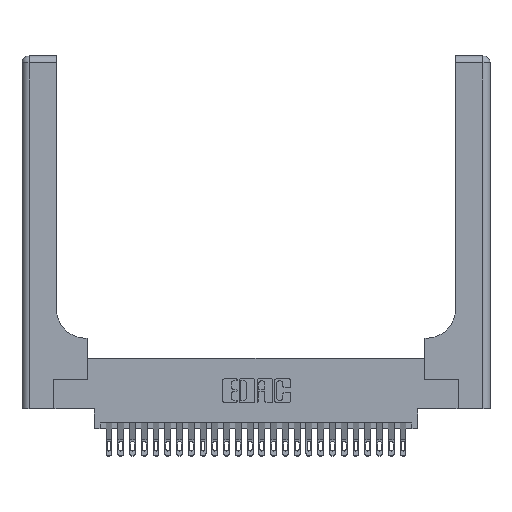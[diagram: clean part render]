
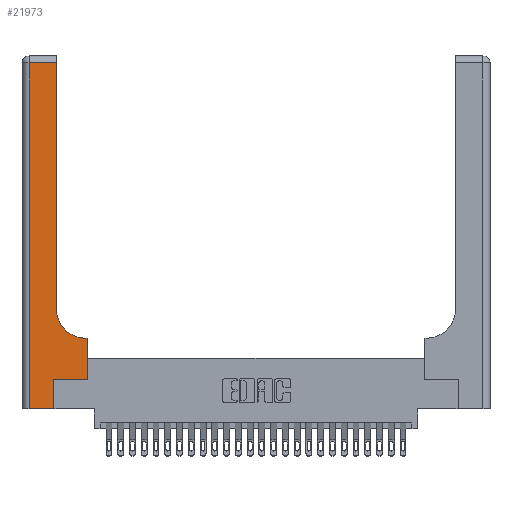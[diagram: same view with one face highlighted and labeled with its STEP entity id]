
A CAD part, top view. The second image highlights one B-rep face of the part: STEP entity #21973.
In plain terms, the highlighted planar face has unit normal (0, 0, 1).
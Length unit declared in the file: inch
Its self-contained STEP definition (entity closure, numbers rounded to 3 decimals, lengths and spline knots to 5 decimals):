
#209 = CARTESIAN_POINT ( 'NONE',  ( 0.269, 0.25, 0.37 ) ) ;
#457 = CARTESIAN_POINT ( 'NONE',  ( 0., 0., 0.37 ) ) ;
#491 = VECTOR ( 'NONE', #25739, 39.37008 ) ;
#656 = CARTESIAN_POINT ( 'NONE',  ( 0., 3., 0.37 ) ) ;
#735 = DIRECTION ( 'NONE',  ( 1., 0., 0. ) ) ;
#740 = DIRECTION ( 'NONE',  ( -1., 0., 0. ) ) ;
#935 = CARTESIAN_POINT ( 'NONE',  ( 0., 2.94, 0.37 ) ) ;
#1166 = LINE ( 'NONE', #1930, #491 ) ;
#1375 = EDGE_CURVE ( 'NONE', #7321, #15064, #19014, .T. ) ;
#1600 = VECTOR ( 'NONE', #14441, 39.37008 ) ;
#1606 = LINE ( 'NONE', #5508, #7385 ) ;
#1655 = EDGE_CURVE ( 'NONE', #11842, #16809, #8755, .T. ) ;
#1930 = CARTESIAN_POINT ( 'NONE',  ( 0.2915, 0.6, 0.37 ) ) ;
#2128 = ORIENTED_EDGE ( 'NONE', *, *, #1655, .T. ) ;
#3147 = ORIENTED_EDGE ( 'NONE', *, *, #14382, .T. ) ;
#3150 = EDGE_CURVE ( 'NONE', #15064, #8248, #1166, .T. ) ;
#3620 = VERTEX_POINT ( 'NONE', #9358 ) ;
#3794 = CARTESIAN_POINT ( 'NONE',  ( 0.2915, 0.85, 0.37 ) ) ;
#3897 = EDGE_CURVE ( 'NONE', #16809, #7321, #12347, .T. ) ;
#5000 = DIRECTION ( 'NONE',  ( 0., 0., -1. ) ) ;
#5508 = CARTESIAN_POINT ( 'NONE',  ( 0.2915, 3., 0.37 ) ) ;
#6095 = ORIENTED_EDGE ( 'NONE', *, *, #3150, .T. ) ;
#6432 = LINE ( 'NONE', #935, #14989 ) ;
#7063 = EDGE_CURVE ( 'NONE', #9543, #10116, #1606, .T. ) ;
#7064 = ORIENTED_EDGE ( 'NONE', *, *, #23813, .T. ) ;
#7321 = VERTEX_POINT ( 'NONE', #18527 ) ;
#7385 = VECTOR ( 'NONE', #20777, 39.37008 ) ;
#7601 = EDGE_LOOP ( 'NONE', ( #12397, #7064, #18103, #3147, #2128, #11591, #24524, #6095, #18890 ) ) ;
#8048 = DIRECTION ( 'NONE',  ( 0., 0., -1. ) ) ;
#8248 = VERTEX_POINT ( 'NONE', #21122 ) ;
#8755 = LINE ( 'NONE', #27491, #1600 ) ;
#9358 = CARTESIAN_POINT ( 'NONE',  ( 0.06, 2.94, 0.37 ) ) ;
#9543 = VERTEX_POINT ( 'NONE', #3794 ) ;
#9610 = VECTOR ( 'NONE', #735, 39.37008 ) ;
#10116 = VERTEX_POINT ( 'NONE', #20019 ) ;
#11130 = CARTESIAN_POINT ( 'NONE',  ( 0.5585, 0.25, 0.37 ) ) ;
#11318 = VERTEX_POINT ( 'NONE', #24661 ) ;
#11519 = CARTESIAN_POINT ( 'NONE',  ( 0.269, 0.25, 0.37 ) ) ;
#11591 = ORIENTED_EDGE ( 'NONE', *, *, #3897, .T. ) ;
#11675 = FACE_OUTER_BOUND ( 'NONE', #7601, .T. ) ;
#11842 = VERTEX_POINT ( 'NONE', #13025 ) ;
#12347 = LINE ( 'NONE', #209, #26332 ) ;
#12397 = ORIENTED_EDGE ( 'NONE', *, *, #7063, .T. ) ;
#12778 = EDGE_CURVE ( 'NONE', #8248, #9543, #13452, .T. ) ;
#13025 = CARTESIAN_POINT ( 'NONE',  ( 0.269, 0., 0.37 ) ) ;
#13452 = CIRCLE ( 'NONE', #27982, 0.25 ) ;
#14382 = EDGE_CURVE ( 'NONE', #11318, #11842, #16123, .T. ) ;
#14441 = DIRECTION ( 'NONE',  ( 0., 1., 0. ) ) ;
#14989 = VECTOR ( 'NONE', #16240, 39.37008 ) ;
#15064 = VERTEX_POINT ( 'NONE', #16015 ) ;
#15498 = VECTOR ( 'NONE', #19671, 39.37008 ) ;
#16015 = CARTESIAN_POINT ( 'NONE',  ( 0.5585, 0.6, 0.37 ) ) ;
#16123 = LINE ( 'NONE', #457, #9610 ) ;
#16240 = DIRECTION ( 'NONE',  ( -1., 0., 0. ) ) ;
#16510 = AXIS2_PLACEMENT_3D ( 'NONE', #656, #5000, #740 ) ;
#16809 = VERTEX_POINT ( 'NONE', #11519 ) ;
#17077 = CARTESIAN_POINT ( 'NONE',  ( 0.5415, 0.85, 0.37 ) ) ;
#17554 = LINE ( 'NONE', #26039, #15498 ) ;
#18103 = ORIENTED_EDGE ( 'NONE', *, *, #21275, .T. ) ;
#18527 = CARTESIAN_POINT ( 'NONE',  ( 0.5585, 0.25, 0.37 ) ) ;
#18890 = ORIENTED_EDGE ( 'NONE', *, *, #12778, .T. ) ;
#19014 = LINE ( 'NONE', #11130, #24116 ) ;
#19181 = DIRECTION ( 'NONE',  ( 1., 0., 0. ) ) ;
#19671 = DIRECTION ( 'NONE',  ( 0., -1., 0. ) ) ;
#20019 = CARTESIAN_POINT ( 'NONE',  ( 0.2915, 2.94, 0.37 ) ) ;
#20777 = DIRECTION ( 'NONE',  ( 0., 1., 0. ) ) ;
#21122 = CARTESIAN_POINT ( 'NONE',  ( 0.5415, 0.6, 0.37 ) ) ;
#21275 = EDGE_CURVE ( 'NONE', #3620, #11318, #17554, .T. ) ;
#21973 = ADVANCED_FACE ( 'NONE', ( #11675 ), #26549, .F. ) ;
#22108 = DIRECTION ( 'NONE',  ( 1., 0., 0. ) ) ;
#23813 = EDGE_CURVE ( 'NONE', #10116, #3620, #6432, .T. ) ;
#24116 = VECTOR ( 'NONE', #24266, 39.37008 ) ;
#24266 = DIRECTION ( 'NONE',  ( 0., 1., 0. ) ) ;
#24524 = ORIENTED_EDGE ( 'NONE', *, *, #1375, .T. ) ;
#24661 = CARTESIAN_POINT ( 'NONE',  ( 0.06, 0., 0.37 ) ) ;
#25739 = DIRECTION ( 'NONE',  ( -1., 0., 0. ) ) ;
#26039 = CARTESIAN_POINT ( 'NONE',  ( 0.06, 3., 0.37 ) ) ;
#26332 = VECTOR ( 'NONE', #22108, 39.37008 ) ;
#26549 = PLANE ( 'NONE',  #16510 ) ;
#27491 = CARTESIAN_POINT ( 'NONE',  ( 0.269, 0., 0.37 ) ) ;
#27982 = AXIS2_PLACEMENT_3D ( 'NONE', #17077, #8048, #19181 ) ;
